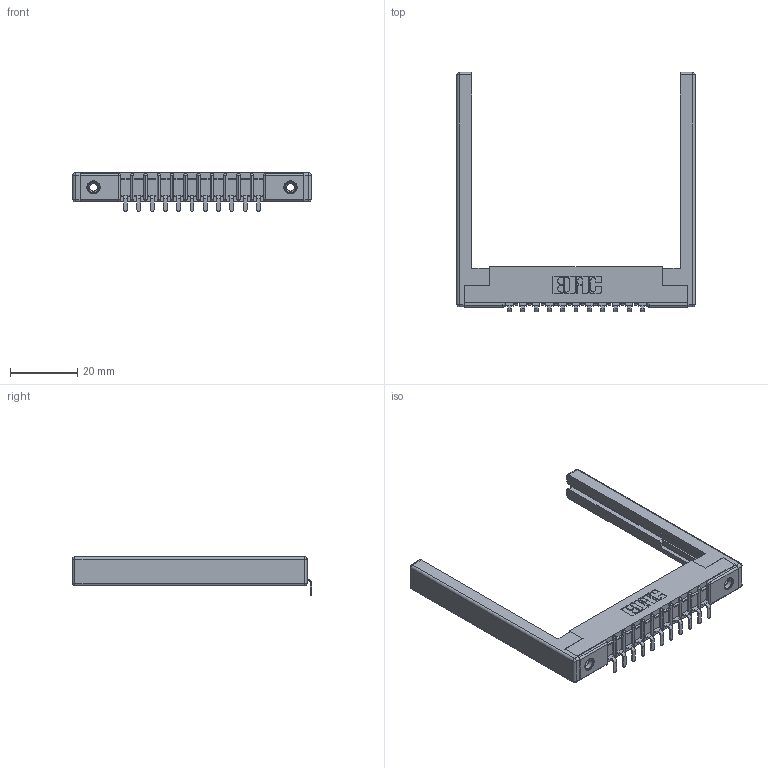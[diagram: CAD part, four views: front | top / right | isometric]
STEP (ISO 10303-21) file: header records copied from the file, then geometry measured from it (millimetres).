
FILE_DESCRIPTION (( 'STEP AP203' ), '1' );
FILE_NAME ('357-011-553-168.STEP', '2019-09-16T18:56:31', ( '' ), ( '' ), 'SwSTEP 2.0', 'SolidWorks 2016', '' );
FILE_SCHEMA (( 'CONFIG_CONTROL_DESIGN' ));
Length unit declared in the file: inch
Products named in the file (5): 307-220-068; 345-250-001_345-250-001-102; 307-290-002_553; 307 Part_.156 Dia Mounting Holes; 357-011-553-168
Assembly tree (16 placements, depth 2):
  357-011-553-168
    307 Part_.156 Dia Mounting Holes
    307-290-002_553  x11
    307-220-068  x2
    345-250-001_345-250-001-102  x2
Bounding box: 71.02 x 71.29 x 11.51 mm (x, y, z)
Volume: 9241.5 mm3; surface area: 11929.3 mm2
Topology: 16 solids, 16 shells, 1142 faces, 3397 edges, 2210 vertices
Faces by surface type: plane 675, cylinder 419, sphere 32, cone 12, torus 4
Entity records: 16865 total; most frequent: CARTESIAN_POINT 2805, ORIENTED_EDGE 2784, DIRECTION 2758, EDGE_CURVE 1392, VECTOR 1048, LINE 1048, VERTEX_POINT 902, AXIS2_PLACEMENT_3D 855
